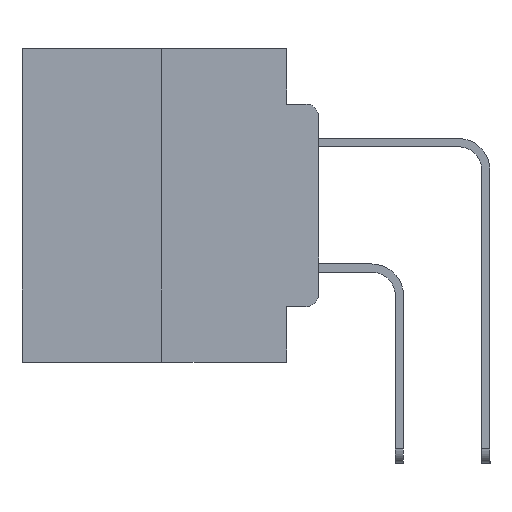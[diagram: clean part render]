
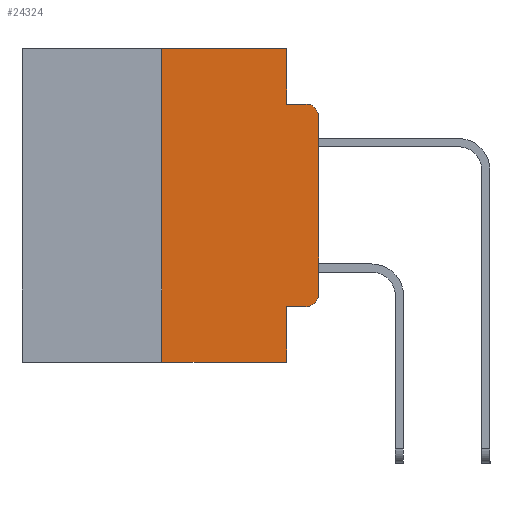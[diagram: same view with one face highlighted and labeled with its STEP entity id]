
A CAD part, left-side view. The second image highlights one B-rep face of the part: STEP entity #24324.
In plain terms, the highlighted planar face has unit normal (-1, 0, 0).
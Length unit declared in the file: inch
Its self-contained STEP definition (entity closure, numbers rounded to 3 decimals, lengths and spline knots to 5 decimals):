
#71 = CIRCLE ( 'NONE', #10487, 0.02 ) ;
#92 = FACE_OUTER_BOUND ( 'NONE', #20595, .T. ) ;
#182 = ORIENTED_EDGE ( 'NONE', *, *, #12856, .F. ) ;
#1135 = CIRCLE ( 'NONE', #7603, 0.02 ) ;
#2257 = CARTESIAN_POINT ( 'NONE',  ( 0., 0.051, 0. ) ) ;
#2428 = CARTESIAN_POINT ( 'NONE',  ( 0., 0., 0. ) ) ;
#2737 = EDGE_CURVE ( 'NONE', #5605, #19048, #71, .T. ) ;
#3376 = DIRECTION ( 'NONE',  ( 0., 0., 1. ) ) ;
#3413 = LINE ( 'NONE', #10025, #18605 ) ;
#4494 = DIRECTION ( 'NONE',  ( 0., 0., -1. ) ) ;
#4524 = EDGE_CURVE ( 'NONE', #26023, #13708, #3413, .T. ) ;
#4679 = CARTESIAN_POINT ( 'NONE',  ( 0., 0.25, -0.5 ) ) ;
#4915 = DIRECTION ( 'NONE',  ( 0., -1., 0. ) ) ;
#5417 = CARTESIAN_POINT ( 'NONE',  ( 0., 0.473, 0. ) ) ;
#5605 = VERTEX_POINT ( 'NONE', #18139 ) ;
#5653 = LINE ( 'NONE', #18930, #27505 ) ;
#5980 = CARTESIAN_POINT ( 'NONE',  ( 0., 0., -0.1085 ) ) ;
#6186 = DIRECTION ( 'NONE',  ( 0., -1., 0. ) ) ;
#6299 = VECTOR ( 'NONE', #21800, 39.37008 ) ;
#6390 = EDGE_CURVE ( 'NONE', #17391, #5605, #5653, .T. ) ;
#6525 = LINE ( 'NONE', #2428, #22167 ) ;
#7463 = ORIENTED_EDGE ( 'NONE', *, *, #2737, .T. ) ;
#7603 = AXIS2_PLACEMENT_3D ( 'NONE', #23764, #11161, #25850 ) ;
#7625 = VECTOR ( 'NONE', #4494, 39.37008 ) ;
#7740 = DIRECTION ( 'NONE',  ( 0., 0., -1. ) ) ;
#8297 = VECTOR ( 'NONE', #4915, 39.37008 ) ;
#8351 = DIRECTION ( 'NONE',  ( 0., 0., -1. ) ) ;
#8458 = ORIENTED_EDGE ( 'NONE', *, *, #19903, .F. ) ;
#8518 = AXIS2_PLACEMENT_3D ( 'NONE', #5417, #20493, #7740 ) ;
#9244 = CARTESIAN_POINT ( 'NONE',  ( 0., 0.473, 0. ) ) ;
#9363 = EDGE_CURVE ( 'NONE', #25180, #15141, #27007, .T. ) ;
#9828 = ORIENTED_EDGE ( 'NONE', *, *, #21386, .F. ) ;
#10025 = CARTESIAN_POINT ( 'NONE',  ( 0., 0.473, -0.5 ) ) ;
#10191 = CARTESIAN_POINT ( 'NONE',  ( 0., 0.051, 0. ) ) ;
#10487 = AXIS2_PLACEMENT_3D ( 'NONE', #21008, #20981, #15504 ) ;
#11161 = DIRECTION ( 'NONE',  ( -1., 0., 0. ) ) ;
#11342 = VERTEX_POINT ( 'NONE', #20876 ) ;
#11398 = LINE ( 'NONE', #15593, #6299 ) ;
#11854 = ORIENTED_EDGE ( 'NONE', *, *, #6390, .T. ) ;
#12435 = CARTESIAN_POINT ( 'NONE',  ( 0., 0.051, -0.0885 ) ) ;
#12856 = EDGE_CURVE ( 'NONE', #17391, #13708, #24516, .T. ) ;
#12872 = ORIENTED_EDGE ( 'NONE', *, *, #18472, .F. ) ;
#13708 = VERTEX_POINT ( 'NONE', #17942 ) ;
#14108 = DIRECTION ( 'NONE',  ( 0., -1., 0. ) ) ;
#14196 = CARTESIAN_POINT ( 'NONE',  ( 0., 0.25, 0. ) ) ;
#15141 = VERTEX_POINT ( 'NONE', #12435 ) ;
#15504 = DIRECTION ( 'NONE',  ( 0., 0., -1. ) ) ;
#15593 = CARTESIAN_POINT ( 'NONE',  ( 0., 0.051, -0.0885 ) ) ;
#15617 = VECTOR ( 'NONE', #3376, 39.37008 ) ;
#16390 = VERTEX_POINT ( 'NONE', #5980 ) ;
#16870 = CARTESIAN_POINT ( 'NONE',  ( 0., 0.051, 0. ) ) ;
#16937 = LINE ( 'NONE', #14196, #15617 ) ;
#17391 = VERTEX_POINT ( 'NONE', #19951 ) ;
#17942 = CARTESIAN_POINT ( 'NONE',  ( 0., 0.051, -0.5 ) ) ;
#18139 = CARTESIAN_POINT ( 'NONE',  ( 0., 0.02, -0.4115 ) ) ;
#18472 = EDGE_CURVE ( 'NONE', #15141, #11342, #11398, .T. ) ;
#18605 = VECTOR ( 'NONE', #14108, 39.37008 ) ;
#18930 = CARTESIAN_POINT ( 'NONE',  ( 0., 0.051, -0.4115 ) ) ;
#19048 = VERTEX_POINT ( 'NONE', #19510 ) ;
#19510 = CARTESIAN_POINT ( 'NONE',  ( 0., 0., -0.3915 ) ) ;
#19676 = DIRECTION ( 'NONE',  ( 0., 0., 1. ) ) ;
#19903 = EDGE_CURVE ( 'NONE', #21478, #25180, #25806, .T. ) ;
#19951 = CARTESIAN_POINT ( 'NONE',  ( 0., 0.051, -0.4115 ) ) ;
#20493 = DIRECTION ( 'NONE',  ( 1., 0., 0. ) ) ;
#20595 = EDGE_LOOP ( 'NONE', ( #22049, #23364, #12872, #24681, #8458, #9828, #21101, #182, #11854, #7463 ) ) ;
#20876 = CARTESIAN_POINT ( 'NONE',  ( 0., 0.02, -0.0885 ) ) ;
#20981 = DIRECTION ( 'NONE',  ( -1., 0., 0. ) ) ;
#21008 = CARTESIAN_POINT ( 'NONE',  ( 0., 0.02, -0.3915 ) ) ;
#21101 = ORIENTED_EDGE ( 'NONE', *, *, #4524, .T. ) ;
#21109 = EDGE_CURVE ( 'NONE', #19048, #16390, #6525, .T. ) ;
#21386 = EDGE_CURVE ( 'NONE', #26023, #21478, #16937, .T. ) ;
#21478 = VERTEX_POINT ( 'NONE', #22935 ) ;
#21503 = VECTOR ( 'NONE', #8351, 39.37008 ) ;
#21800 = DIRECTION ( 'NONE',  ( 0., -1., 0. ) ) ;
#22049 = ORIENTED_EDGE ( 'NONE', *, *, #21109, .T. ) ;
#22167 = VECTOR ( 'NONE', #19676, 39.37008 ) ;
#22482 = PLANE ( 'NONE',  #8518 ) ;
#22935 = CARTESIAN_POINT ( 'NONE',  ( 0., 0.25, 0. ) ) ;
#23364 = ORIENTED_EDGE ( 'NONE', *, *, #24046, .T. ) ;
#23764 = CARTESIAN_POINT ( 'NONE',  ( 0., 0.02, -0.1085 ) ) ;
#24046 = EDGE_CURVE ( 'NONE', #16390, #11342, #1135, .T. ) ;
#24324 = ADVANCED_FACE ( 'NONE', ( #92 ), #22482, .F. ) ;
#24516 = LINE ( 'NONE', #2257, #7625 ) ;
#24681 = ORIENTED_EDGE ( 'NONE', *, *, #9363, .F. ) ;
#25180 = VERTEX_POINT ( 'NONE', #10191 ) ;
#25806 = LINE ( 'NONE', #9244, #8297 ) ;
#25850 = DIRECTION ( 'NONE',  ( 0., 0., -1. ) ) ;
#26023 = VERTEX_POINT ( 'NONE', #4679 ) ;
#27007 = LINE ( 'NONE', #16870, #21503 ) ;
#27505 = VECTOR ( 'NONE', #6186, 39.37008 ) ;
